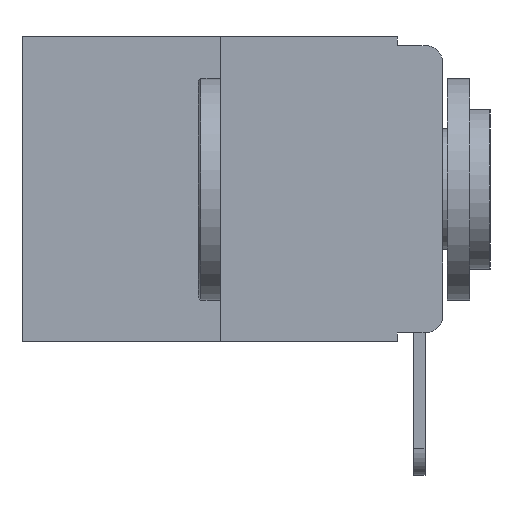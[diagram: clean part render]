
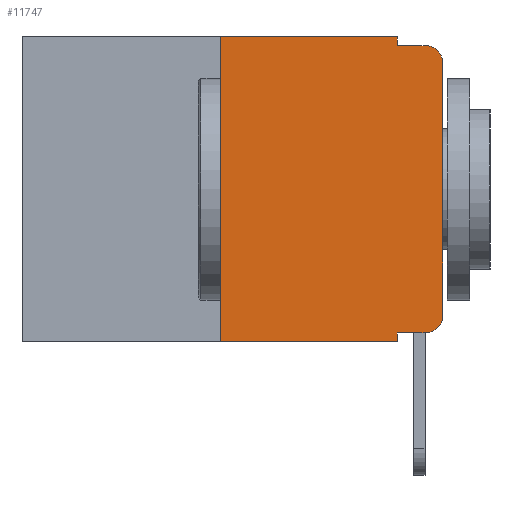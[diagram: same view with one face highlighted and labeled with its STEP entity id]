
A CAD part, left-side view. The second image highlights one B-rep face of the part: STEP entity #11747.
In plain terms, the highlighted planar face has unit normal (-1, 0, 0).
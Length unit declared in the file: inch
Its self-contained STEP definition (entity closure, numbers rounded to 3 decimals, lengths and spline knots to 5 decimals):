
#37 = LINE ( 'NONE', #16977, #16768 ) ;
#778 = VERTEX_POINT ( 'NONE', #4313 ) ;
#1343 = ORIENTED_EDGE ( 'NONE', *, *, #12439, .F. ) ;
#2377 = CARTESIAN_POINT ( 'NONE',  ( 0., 0.051, 0. ) ) ;
#2566 = VECTOR ( 'NONE', #7402, 39.37008 ) ;
#3134 = ORIENTED_EDGE ( 'NONE', *, *, #12664, .T. ) ;
#3151 = EDGE_CURVE ( 'NONE', #7751, #12966, #3260, .T. ) ;
#3237 = VERTEX_POINT ( 'NONE', #6782 ) ;
#3260 = LINE ( 'NONE', #19802, #14390 ) ;
#3511 = LINE ( 'NONE', #18346, #2566 ) ;
#3516 = EDGE_CURVE ( 'NONE', #8772, #13823, #17167, .T. ) ;
#3598 = DIRECTION ( 'NONE',  ( 0., -1., 0. ) ) ;
#4200 = AXIS2_PLACEMENT_3D ( 'NONE', #7453, #14876, #22297 ) ;
#4313 = CARTESIAN_POINT ( 'NONE',  ( 0., 0.02, -0.01 ) ) ;
#4707 = VECTOR ( 'NONE', #11244, 39.37008 ) ;
#5158 = VERTEX_POINT ( 'NONE', #10140 ) ;
#6233 = EDGE_CURVE ( 'NONE', #13823, #22413, #11616, .T. ) ;
#6660 = AXIS2_PLACEMENT_3D ( 'NONE', #20774, #11766, #11530 ) ;
#6755 = EDGE_CURVE ( 'NONE', #22413, #778, #9260, .T. ) ;
#6782 = CARTESIAN_POINT ( 'NONE',  ( 0., 0.051, -0.01 ) ) ;
#7019 = DIRECTION ( 'NONE',  ( 0., 0., 1. ) ) ;
#7402 = DIRECTION ( 'NONE',  ( 0., -1., 0. ) ) ;
#7453 = CARTESIAN_POINT ( 'NONE',  ( 0., 0.02, -0.03 ) ) ;
#7481 = CARTESIAN_POINT ( 'NONE',  ( 0., 0., 0. ) ) ;
#7751 = VERTEX_POINT ( 'NONE', #21217 ) ;
#7935 = ORIENTED_EDGE ( 'NONE', *, *, #14356, .F. ) ;
#8011 = DIRECTION ( 'NONE',  ( 0., 0., -1. ) ) ;
#8767 = LINE ( 'NONE', #16415, #19935 ) ;
#8772 = VERTEX_POINT ( 'NONE', #23715 ) ;
#9014 = DIRECTION ( 'NONE',  ( 0., 0., -1. ) ) ;
#9260 = CIRCLE ( 'NONE', #4200, 0.02 ) ;
#10019 = EDGE_CURVE ( 'NONE', #17953, #5158, #12876, .T. ) ;
#10105 = LINE ( 'NONE', #23129, #17096 ) ;
#10140 = CARTESIAN_POINT ( 'NONE',  ( 0., 0.25, 0. ) ) ;
#10167 = ORIENTED_EDGE ( 'NONE', *, *, #6233, .T. ) ;
#10464 = DIRECTION ( 'NONE',  ( 1., 0., 0. ) ) ;
#10807 = DIRECTION ( 'NONE',  ( 0., 0., -1. ) ) ;
#10903 = AXIS2_PLACEMENT_3D ( 'NONE', #19834, #10464, #9014 ) ;
#11244 = DIRECTION ( 'NONE',  ( 0., 0., 1. ) ) ;
#11530 = DIRECTION ( 'NONE',  ( 0., 0., -1. ) ) ;
#11616 = LINE ( 'NONE', #7481, #4707 ) ;
#11649 = EDGE_CURVE ( 'NONE', #3237, #778, #10105, .T. ) ;
#11747 = ADVANCED_FACE ( 'NONE', ( #14615 ), #12679, .F. ) ;
#11766 = DIRECTION ( 'NONE',  ( -1., 0., 0. ) ) ;
#11942 = CARTESIAN_POINT ( 'NONE',  ( 0., 0.051, 0. ) ) ;
#12439 = EDGE_CURVE ( 'NONE', #21655, #3237, #22947, .T. ) ;
#12643 = CARTESIAN_POINT ( 'NONE',  ( 0., 0.25, 0. ) ) ;
#12664 = EDGE_CURVE ( 'NONE', #17953, #12966, #37, .T. ) ;
#12679 = PLANE ( 'NONE',  #10903 ) ;
#12876 = LINE ( 'NONE', #12643, #17112 ) ;
#12909 = ORIENTED_EDGE ( 'NONE', *, *, #3516, .T. ) ;
#12966 = VERTEX_POINT ( 'NONE', #13915 ) ;
#13823 = VERTEX_POINT ( 'NONE', #16130 ) ;
#13890 = DIRECTION ( 'NONE',  ( 0., -1., 0. ) ) ;
#13915 = CARTESIAN_POINT ( 'NONE',  ( 0., 0.051, -0.343 ) ) ;
#14238 = DIRECTION ( 'NONE',  ( 0., -1., 0. ) ) ;
#14356 = EDGE_CURVE ( 'NONE', #5158, #21655, #8767, .T. ) ;
#14390 = VECTOR ( 'NONE', #10807, 39.37008 ) ;
#14615 = FACE_OUTER_BOUND ( 'NONE', #21980, .T. ) ;
#14792 = CARTESIAN_POINT ( 'NONE',  ( 0., 0.25, -0.343 ) ) ;
#14876 = DIRECTION ( 'NONE',  ( -1., 0., 0. ) ) ;
#15660 = ORIENTED_EDGE ( 'NONE', *, *, #23869, .T. ) ;
#16130 = CARTESIAN_POINT ( 'NONE',  ( 0., 0., -0.313 ) ) ;
#16323 = ORIENTED_EDGE ( 'NONE', *, *, #10019, .F. ) ;
#16415 = CARTESIAN_POINT ( 'NONE',  ( 0., 0.473, 0. ) ) ;
#16768 = VECTOR ( 'NONE', #3598, 39.37008 ) ;
#16977 = CARTESIAN_POINT ( 'NONE',  ( 0., 0.473, -0.343 ) ) ;
#17096 = VECTOR ( 'NONE', #13890, 39.37008 ) ;
#17112 = VECTOR ( 'NONE', #7019, 39.37008 ) ;
#17131 = VECTOR ( 'NONE', #8011, 39.37008 ) ;
#17167 = CIRCLE ( 'NONE', #6660, 0.02 ) ;
#17624 = CARTESIAN_POINT ( 'NONE',  ( 0., 0., -0.03 ) ) ;
#17953 = VERTEX_POINT ( 'NONE', #14792 ) ;
#18346 = CARTESIAN_POINT ( 'NONE',  ( 0., 0.051, -0.333 ) ) ;
#18663 = ORIENTED_EDGE ( 'NONE', *, *, #6755, .T. ) ;
#19676 = ORIENTED_EDGE ( 'NONE', *, *, #11649, .F. ) ;
#19802 = CARTESIAN_POINT ( 'NONE',  ( 0., 0.051, 0. ) ) ;
#19834 = CARTESIAN_POINT ( 'NONE',  ( 0., 0.473, 0. ) ) ;
#19935 = VECTOR ( 'NONE', #14238, 39.37008 ) ;
#20774 = CARTESIAN_POINT ( 'NONE',  ( 0., 0.02, -0.313 ) ) ;
#20853 = ORIENTED_EDGE ( 'NONE', *, *, #3151, .F. ) ;
#21217 = CARTESIAN_POINT ( 'NONE',  ( 0., 0.051, -0.333 ) ) ;
#21655 = VERTEX_POINT ( 'NONE', #11942 ) ;
#21980 = EDGE_LOOP ( 'NONE', ( #10167, #18663, #19676, #1343, #7935, #16323, #3134, #20853, #15660, #12909 ) ) ;
#22297 = DIRECTION ( 'NONE',  ( 0., 0., -1. ) ) ;
#22413 = VERTEX_POINT ( 'NONE', #17624 ) ;
#22947 = LINE ( 'NONE', #2377, #17131 ) ;
#23129 = CARTESIAN_POINT ( 'NONE',  ( 0., 0.051, -0.01 ) ) ;
#23715 = CARTESIAN_POINT ( 'NONE',  ( 0., 0.02, -0.333 ) ) ;
#23869 = EDGE_CURVE ( 'NONE', #7751, #8772, #3511, .T. ) ;
